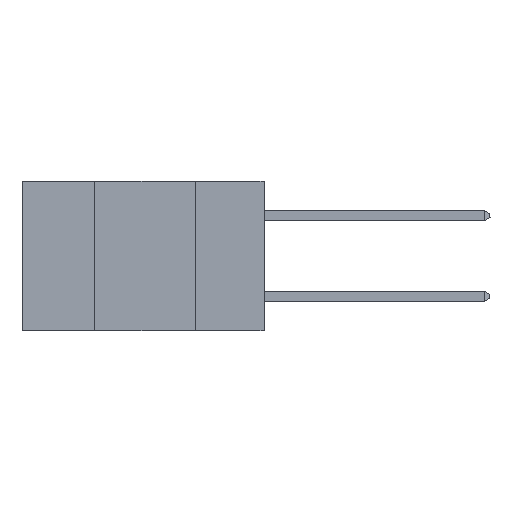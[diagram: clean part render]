
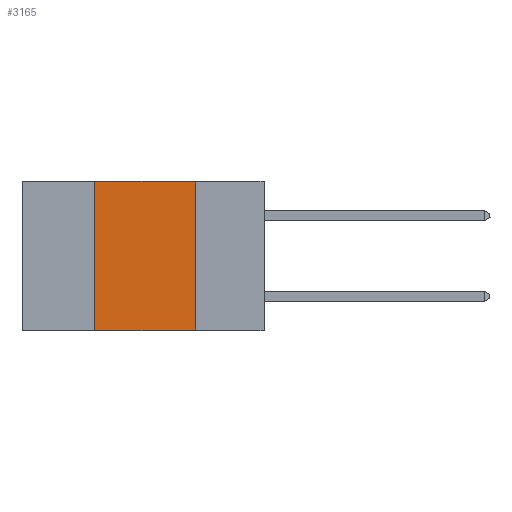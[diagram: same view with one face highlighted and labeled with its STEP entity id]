
A CAD part, left-side view. The second image highlights one B-rep face of the part: STEP entity #3165.
In plain terms, the highlighted planar face has unit normal (-1, 0, 0).
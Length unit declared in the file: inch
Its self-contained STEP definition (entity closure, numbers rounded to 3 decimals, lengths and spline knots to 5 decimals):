
#1189 = CARTESIAN_POINT ( 'NONE',  ( 0., 0.42, 0. ) ) ;
#2438 = FACE_OUTER_BOUND ( 'NONE', #9909, .T. ) ;
#2822 = EDGE_CURVE ( 'NONE', #24090, #11078, #14339, .T. ) ;
#2867 = VERTEX_POINT ( 'NONE', #14327 ) ;
#3165 = ADVANCED_FACE ( 'NONE', ( #2438 ), #3647, .F. ) ;
#3647 = PLANE ( 'NONE',  #3883 ) ;
#3883 = AXIS2_PLACEMENT_3D ( 'NONE', #25494, #6018, #10108 ) ;
#4849 = ORIENTED_EDGE ( 'NONE', *, *, #7407, .F. ) ;
#6018 = DIRECTION ( 'NONE',  ( 1., 0., 0. ) ) ;
#7361 = CARTESIAN_POINT ( 'NONE',  ( 0., 0.6, 0. ) ) ;
#7407 = EDGE_CURVE ( 'NONE', #11078, #2867, #20091, .T. ) ;
#8599 = ORIENTED_EDGE ( 'NONE', *, *, #19805, .F. ) ;
#9909 = EDGE_LOOP ( 'NONE', ( #8599, #4849, #27872, #12578 ) ) ;
#10108 = DIRECTION ( 'NONE',  ( 0., 0., -1. ) ) ;
#10467 = VECTOR ( 'NONE', #22183, 39.37008 ) ;
#11078 = VERTEX_POINT ( 'NONE', #1189 ) ;
#11324 = CARTESIAN_POINT ( 'NONE',  ( 0., 0.6, -0.37 ) ) ;
#12041 = DIRECTION ( 'NONE',  ( 0., 0., 1. ) ) ;
#12578 = ORIENTED_EDGE ( 'NONE', *, *, #13602, .T. ) ;
#12591 = CARTESIAN_POINT ( 'NONE',  ( 0., 0.17, 0. ) ) ;
#13602 = EDGE_CURVE ( 'NONE', #24090, #20766, #21707, .T. ) ;
#14327 = CARTESIAN_POINT ( 'NONE',  ( 0., 0.17, 0. ) ) ;
#14339 = LINE ( 'NONE', #25156, #25565 ) ;
#16222 = VECTOR ( 'NONE', #27793, 39.37008 ) ;
#16549 = LINE ( 'NONE', #12591, #16222 ) ;
#19805 = EDGE_CURVE ( 'NONE', #2867, #20766, #16549, .T. ) ;
#20091 = LINE ( 'NONE', #7361, #22821 ) ;
#20242 = CARTESIAN_POINT ( 'NONE',  ( 0., 0.17, -0.37 ) ) ;
#20766 = VERTEX_POINT ( 'NONE', #20242 ) ;
#21707 = LINE ( 'NONE', #11324, #10467 ) ;
#22183 = DIRECTION ( 'NONE',  ( 0., -1., 0. ) ) ;
#22567 = DIRECTION ( 'NONE',  ( 0., -1., 0. ) ) ;
#22821 = VECTOR ( 'NONE', #22567, 39.37008 ) ;
#24090 = VERTEX_POINT ( 'NONE', #25301 ) ;
#25156 = CARTESIAN_POINT ( 'NONE',  ( 0., 0.42, 0. ) ) ;
#25301 = CARTESIAN_POINT ( 'NONE',  ( 0., 0.42, -0.37 ) ) ;
#25494 = CARTESIAN_POINT ( 'NONE',  ( 0., 0.6, 0. ) ) ;
#25565 = VECTOR ( 'NONE', #12041, 39.37008 ) ;
#27793 = DIRECTION ( 'NONE',  ( 0., 0., -1. ) ) ;
#27872 = ORIENTED_EDGE ( 'NONE', *, *, #2822, .F. ) ;
